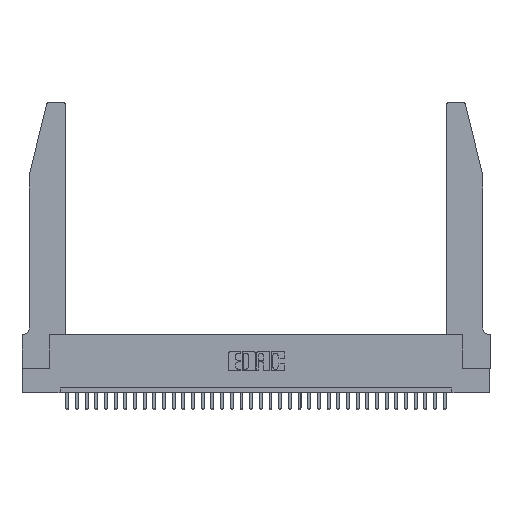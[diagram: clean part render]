
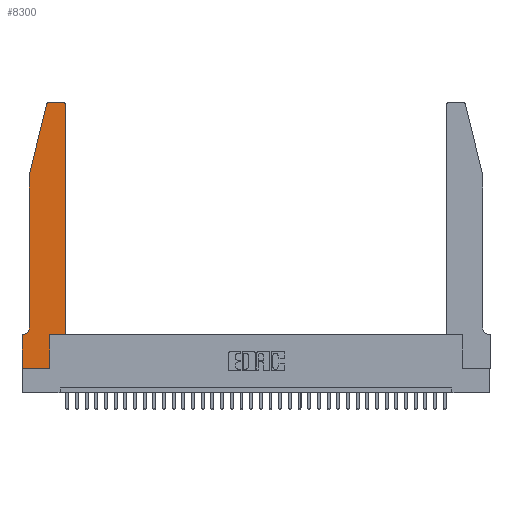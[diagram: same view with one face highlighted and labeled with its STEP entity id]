
A CAD part, top view. The second image highlights one B-rep face of the part: STEP entity #8300.
In plain terms, the highlighted planar face has unit normal (0, 0, 1).
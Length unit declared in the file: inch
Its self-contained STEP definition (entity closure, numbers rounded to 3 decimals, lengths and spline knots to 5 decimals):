
#963 = ORIENTED_EDGE ( 'NONE', *, *, #14655, .T. ) ;
#1101 = CARTESIAN_POINT ( 'NONE',  ( 0.284, 2.75, 0.37 ) ) ;
#1251 = CARTESIAN_POINT ( 'NONE',  ( 0.4505, 2.72, 0.37 ) ) ;
#1403 = ORIENTED_EDGE ( 'NONE', *, *, #29812, .T. ) ;
#1502 = CARTESIAN_POINT ( 'NONE',  ( 0.4205, 2.75, 0.37 ) ) ;
#1547 = LINE ( 'NONE', #13266, #29649 ) ;
#1951 = LINE ( 'NONE', #21476, #7929 ) ;
#2274 = CARTESIAN_POINT ( 'NONE',  ( 0.4505, 0.35, 0.37 ) ) ;
#2304 = CARTESIAN_POINT ( 'NONE',  ( 0.25487, 2.72718, 0.37 ) ) ;
#3023 = ORIENTED_EDGE ( 'NONE', *, *, #23746, .T. ) ;
#3051 = PLANE ( 'NONE',  #18924 ) ;
#3438 = CARTESIAN_POINT ( 'NONE',  ( 0.0055, 0.42, 0.37 ) ) ;
#4122 = VERTEX_POINT ( 'NONE', #30124 ) ;
#4417 = EDGE_CURVE ( 'NONE', #21981, #7422, #1547, .T. ) ;
#4944 = VECTOR ( 'NONE', #11209, 39.37008 ) ;
#6709 = CIRCLE ( 'NONE', #28209, 0.07 ) ;
#6738 = ORIENTED_EDGE ( 'NONE', *, *, #13370, .T. ) ;
#6796 = VECTOR ( 'NONE', #7550, 39.37008 ) ;
#7315 = DIRECTION ( 'NONE',  ( 0., 0., 1. ) ) ;
#7422 = VERTEX_POINT ( 'NONE', #23651 ) ;
#7503 = VERTEX_POINT ( 'NONE', #22037 ) ;
#7550 = DIRECTION ( 'NONE',  ( 0., -1., 0. ) ) ;
#7629 = CARTESIAN_POINT ( 'NONE',  ( 0.2865, 0.35, 0.37 ) ) ;
#7840 = EDGE_CURVE ( 'NONE', #7422, #4122, #19534, .T. ) ;
#7929 = VECTOR ( 'NONE', #35121, 39.37008 ) ;
#8083 = ORIENTED_EDGE ( 'NONE', *, *, #32371, .T. ) ;
#8235 = VECTOR ( 'NONE', #13937, 39.37008 ) ;
#8300 = ADVANCED_FACE ( 'NONE', ( #24630 ), #3051, .T. ) ;
#8592 = VECTOR ( 'NONE', #24680, 39.37008 ) ;
#8764 = LINE ( 'NONE', #27513, #4944 ) ;
#9339 = LINE ( 'NONE', #32153, #6796 ) ;
#9346 = CARTESIAN_POINT ( 'NONE',  ( 0.0755, 0.42, 0.37 ) ) ;
#9685 = LINE ( 'NONE', #29471, #16880 ) ;
#10241 = DIRECTION ( 'NONE',  ( -1., 0., 0. ) ) ;
#11209 = DIRECTION ( 'NONE',  ( -1., 0., 0. ) ) ;
#11285 = ORIENTED_EDGE ( 'NONE', *, *, #19187, .T. ) ;
#11598 = ORIENTED_EDGE ( 'NONE', *, *, #26499, .T. ) ;
#11913 = DIRECTION ( 'NONE',  ( -1., 0., 0. ) ) ;
#12299 = CIRCLE ( 'NONE', #25760, 0.03 ) ;
#12781 = DIRECTION ( 'NONE',  ( 1., 0., 0. ) ) ;
#13233 = ORIENTED_EDGE ( 'NONE', *, *, #15636, .T. ) ;
#13266 = CARTESIAN_POINT ( 'NONE',  ( 0., 0., 0.37 ) ) ;
#13370 = EDGE_CURVE ( 'NONE', #7503, #30030, #9685, .T. ) ;
#13937 = DIRECTION ( 'NONE',  ( -0.239, -0.971, 0. ) ) ;
#14655 = EDGE_CURVE ( 'NONE', #31179, #23109, #23196, .T. ) ;
#14919 = VECTOR ( 'NONE', #26999, 39.37008 ) ;
#15623 = CARTESIAN_POINT ( 'NONE',  ( 0., 0.35, 0.37 ) ) ;
#15636 = EDGE_CURVE ( 'NONE', #4122, #27051, #23131, .T. ) ;
#16279 = VERTEX_POINT ( 'NONE', #9346 ) ;
#16367 = CARTESIAN_POINT ( 'NONE',  ( 0., 0., 0.37 ) ) ;
#16643 = LINE ( 'NONE', #16367, #8592 ) ;
#16852 = CARTESIAN_POINT ( 'NONE',  ( 0., 0., 0.37 ) ) ;
#16880 = VECTOR ( 'NONE', #10241, 39.37008 ) ;
#17236 = CARTESIAN_POINT ( 'NONE',  ( 0.4205, 2.72, 0.37 ) ) ;
#17443 = ORIENTED_EDGE ( 'NONE', *, *, #21451, .T. ) ;
#17461 = EDGE_LOOP ( 'NONE', ( #11285, #963, #17443, #3023, #1403, #6738, #11598, #31285, #18152, #13233, #27859, #8083 ) ) ;
#17472 = DIRECTION ( 'NONE',  ( 1., 0., 0. ) ) ;
#18152 = ORIENTED_EDGE ( 'NONE', *, *, #7840, .T. ) ;
#18924 = AXIS2_PLACEMENT_3D ( 'NONE', #22119, #27588, #24515 ) ;
#19006 = EDGE_CURVE ( 'NONE', #27051, #35083, #1951, .T. ) ;
#19187 = EDGE_CURVE ( 'NONE', #26207, #31179, #8764, .T. ) ;
#19534 = LINE ( 'NONE', #7629, #14919 ) ;
#21451 = EDGE_CURVE ( 'NONE', #23109, #22028, #21849, .T. ) ;
#21476 = CARTESIAN_POINT ( 'NONE',  ( 0.4505, 0.35, 0.37 ) ) ;
#21849 = LINE ( 'NONE', #22137, #8235 ) ;
#21981 = VERTEX_POINT ( 'NONE', #16852 ) ;
#22028 = VERTEX_POINT ( 'NONE', #27674 ) ;
#22037 = CARTESIAN_POINT ( 'NONE',  ( 0.0055, 0.35, 0.37 ) ) ;
#22119 = CARTESIAN_POINT ( 'NONE',  ( 0., 0.35, 0.37 ) ) ;
#22137 = CARTESIAN_POINT ( 'NONE',  ( 0.0755, 2., 0.37 ) ) ;
#22717 = DIRECTION ( 'NONE',  ( 0., 0., 1. ) ) ;
#23109 = VERTEX_POINT ( 'NONE', #2304 ) ;
#23131 = LINE ( 'NONE', #25548, #31665 ) ;
#23196 = CIRCLE ( 'NONE', #24497, 0.03 ) ;
#23651 = CARTESIAN_POINT ( 'NONE',  ( 0.2865, 0., 0.37 ) ) ;
#23746 = EDGE_CURVE ( 'NONE', #22028, #16279, #9339, .T. ) ;
#24497 = AXIS2_PLACEMENT_3D ( 'NONE', #26103, #7315, #12781 ) ;
#24515 = DIRECTION ( 'NONE',  ( 1., 0., 0. ) ) ;
#24630 = FACE_OUTER_BOUND ( 'NONE', #17461, .T. ) ;
#24680 = DIRECTION ( 'NONE',  ( 0., -1., 0. ) ) ;
#25548 = CARTESIAN_POINT ( 'NONE',  ( 0.4505, 0.35, 0.37 ) ) ;
#25760 = AXIS2_PLACEMENT_3D ( 'NONE', #17236, #22717, #17472 ) ;
#26103 = CARTESIAN_POINT ( 'NONE',  ( 0.284, 2.72, 0.37 ) ) ;
#26207 = VERTEX_POINT ( 'NONE', #1502 ) ;
#26499 = EDGE_CURVE ( 'NONE', #30030, #21981, #16643, .T. ) ;
#26931 = DIRECTION ( 'NONE',  ( 1., 0., 0. ) ) ;
#26999 = DIRECTION ( 'NONE',  ( 0., 1., 0. ) ) ;
#27051 = VERTEX_POINT ( 'NONE', #2274 ) ;
#27513 = CARTESIAN_POINT ( 'NONE',  ( 0.2605, 2.75, 0.37 ) ) ;
#27588 = DIRECTION ( 'NONE',  ( 0., 0., 1. ) ) ;
#27674 = CARTESIAN_POINT ( 'NONE',  ( 0.0755, 2., 0.37 ) ) ;
#27859 = ORIENTED_EDGE ( 'NONE', *, *, #19006, .T. ) ;
#28199 = DIRECTION ( 'NONE',  ( 0., 0., -1. ) ) ;
#28209 = AXIS2_PLACEMENT_3D ( 'NONE', #3438, #28199, #11913 ) ;
#29471 = CARTESIAN_POINT ( 'NONE',  ( 0.0755, 0.35, 0.37 ) ) ;
#29649 = VECTOR ( 'NONE', #26931, 39.37008 ) ;
#29812 = EDGE_CURVE ( 'NONE', #16279, #7503, #6709, .T. ) ;
#30030 = VERTEX_POINT ( 'NONE', #15623 ) ;
#30124 = CARTESIAN_POINT ( 'NONE',  ( 0.2865, 0.35, 0.37 ) ) ;
#31179 = VERTEX_POINT ( 'NONE', #1101 ) ;
#31285 = ORIENTED_EDGE ( 'NONE', *, *, #4417, .T. ) ;
#31665 = VECTOR ( 'NONE', #33522, 39.37008 ) ;
#32153 = CARTESIAN_POINT ( 'NONE',  ( 0.0755, 2., 0.37 ) ) ;
#32371 = EDGE_CURVE ( 'NONE', #35083, #26207, #12299, .T. ) ;
#33522 = DIRECTION ( 'NONE',  ( 1., 0., 0. ) ) ;
#35083 = VERTEX_POINT ( 'NONE', #1251 ) ;
#35121 = DIRECTION ( 'NONE',  ( 0., 1., 0. ) ) ;
